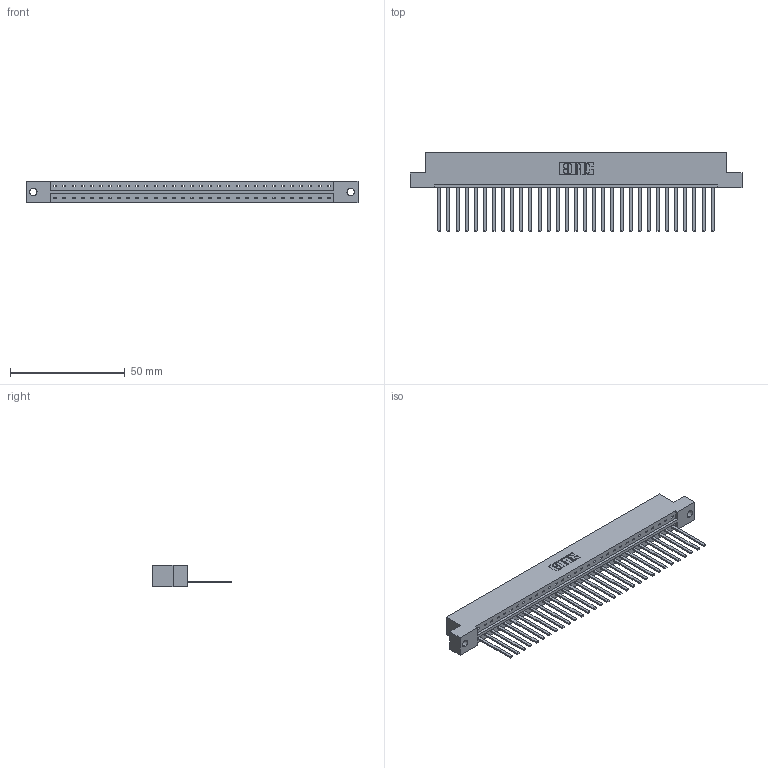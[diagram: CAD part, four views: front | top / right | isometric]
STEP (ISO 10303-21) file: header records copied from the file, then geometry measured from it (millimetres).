
FILE_DESCRIPTION (( 'STEP AP203' ), '1' );
FILE_NAME ('833-031-544-102.STEP', '2020-06-02T15:51:05', ( '' ), ( '' ), 'SwSTEP 2.0', 'SolidWorks 2020', '' );
FILE_SCHEMA (( 'CONFIG_CONTROL_DESIGN' ));
Length unit declared in the file: inch
Products named in the file (3): 345-292-001_345-293-144; 833-031-544-102; 833 Part_Flush - .128 Dia
Assembly tree (32 placements, depth 2):
  833-031-544-102
    833 Part_Flush - .128 Dia
    345-292-001_345-293-144  x31
Bounding box: 144.37 x 34.3 x 9.4 mm (x, y, z)
Volume: 14755.8 mm3; surface area: 16788.7 mm2
Topology: 32 solids, 32 shells, 1726 faces, 5209 edges, 3430 vertices
Faces by surface type: plane 1248, cylinder 478
Entity records: 20193 total; most frequent: CARTESIAN_POINT 3491, ORIENTED_EDGE 3458, DIRECTION 2963, EDGE_CURVE 1729, VECTOR 1605, LINE 1605, VERTEX_POINT 1150, AXIS2_PLACEMENT_3D 679
